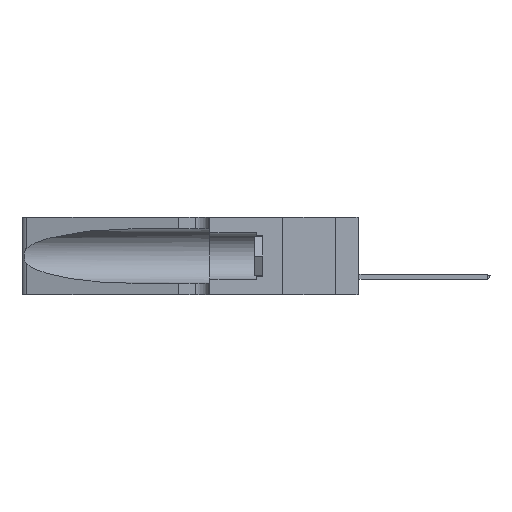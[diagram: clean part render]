
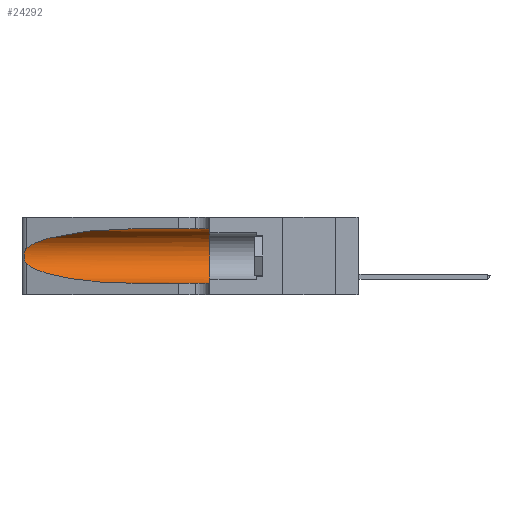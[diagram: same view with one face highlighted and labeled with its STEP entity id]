
A CAD part, left-side view. The second image highlights one B-rep face of the part: STEP entity #24292.
In plain terms, the highlighted cylindrical face has radius 3.308 mm (diameter 6.617 mm), a partial arc.
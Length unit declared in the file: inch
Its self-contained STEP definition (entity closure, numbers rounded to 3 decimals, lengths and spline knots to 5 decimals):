
#578 = ORIENTED_EDGE ( 'NONE', *, *, #11066, .F. ) ;
#1129 = VERTEX_POINT ( 'NONE', #12035 ) ;
#1414 = CARTESIAN_POINT ( 'NONE',  ( 0.25487, 1.22718, 0.14631 ) ) ;
#2001 = EDGE_CURVE ( 'NONE', #14737, #4103, #17094, .T. ) ;
#2032 = ORIENTED_EDGE ( 'NONE', *, *, #13607, .F. ) ;
#2352 = CARTESIAN_POINT ( 'NONE',  ( 0.1305, 0.72297, 0.31525 ) ) ;
#2477 = CARTESIAN_POINT ( 'NONE',  ( 0.1305, 1.61858, 0.31525 ) ) ;
#2659 = CARTESIAN_POINT ( 'NONE',  ( 0.25487, 1.22718, 0.22369 ) ) ;
#2972 = VERTEX_POINT ( 'NONE', #2352 ) ;
#3189 = CARTESIAN_POINT ( 'NONE',  ( 0.25487, 1.22718, 0.22369 ) ) ;
#3365 = CARTESIAN_POINT ( 'NONE',  ( 0.2373, 1.15595, 0.28018 ) ) ;
#3425 = CARTESIAN_POINT ( 'NONE',  ( 0.26075, 1.23896, 0.19203 ) ) ;
#3969 = AXIS2_PLACEMENT_3D ( 'NONE', #17605, #17777, #21797 ) ;
#4103 = VERTEX_POINT ( 'NONE', #18548 ) ;
#4219 = LINE ( 'NONE', #2477, #13924 ) ;
#4576 = EDGE_CURVE ( 'NONE', #2972, #10317, #12386, .T. ) ;
#5140 = CARTESIAN_POINT ( 'NONE',  ( 0.25787, 1.23484, 0.2124 ) ) ;
#5484 = CARTESIAN_POINT ( 'NONE',  ( 0.25487, 1.22718, 0.22369 ) ) ;
#5538 = EDGE_CURVE ( 'NONE', #10317, #14737, #11249, .T. ) ;
#5572 = ORIENTED_EDGE ( 'NONE', *, *, #2001, .T. ) ;
#7021 = ORIENTED_EDGE ( 'NONE', *, *, #15841, .T. ) ;
#7035 = CARTESIAN_POINT ( 'NONE',  ( 0.26017, 1.23833, 0.17102 ) ) ;
#7120 = CARTESIAN_POINT ( 'NONE',  ( 0.26018, 1.23835, 0.19895 ) ) ;
#7374 = CARTESIAN_POINT ( 'NONE',  ( 0.26075, 1.23896, 0.178 ) ) ;
#7436 = CARTESIAN_POINT ( 'NONE',  ( 0.1305, 0.35, 0.05475 ) ) ;
#7580 = FACE_OUTER_BOUND ( 'NONE', #13297, .T. ) ;
#8083 = ORIENTED_EDGE ( 'NONE', *, *, #4576, .T. ) ;
#8667 = LINE ( 'NONE', #12979, #9627 ) ;
#9627 = VECTOR ( 'NONE', #11195, 39.37008 ) ;
#10317 = VERTEX_POINT ( 'NONE', #2659 ) ;
#11066 = EDGE_CURVE ( 'NONE', #2972, #1129, #4219, .T. ) ;
#11195 = DIRECTION ( 'NONE',  ( 0., -1., 0. ) ) ;
#11231 = CARTESIAN_POINT ( 'NONE',  ( 0.25639, 1.23186, 0.15144 ) ) ;
#11249 = B_SPLINE_CURVE_WITH_KNOTS ( 'NONE', 3,
 ( #5484, #19344, #15117, #5140, #11403, #7120, #3425, #7374, #7035, #21347, #11323, #11231, #17424, #1414 ),
 .UNSPECIFIED., .F., .F.,
 ( 4, 2, 2, 2, 2, 2, 4 ),
 ( 0., 0.00027, 0.00053, 0.00107, 0.0016, 0.00187, 0.00214 ),
 .UNSPECIFIED. ) ;
#11283 = ORIENTED_EDGE ( 'NONE', *, *, #5538, .T. ) ;
#11323 = CARTESIAN_POINT ( 'NONE',  ( 0.25789, 1.23486, 0.15765 ) ) ;
#11403 = CARTESIAN_POINT ( 'NONE',  ( 0.25854, 1.2359, 0.20912 ) ) ;
#11491 = CARTESIAN_POINT ( 'NONE',  ( 0.25487, 1.22718, 0.14631 ) ) ;
#12035 = CARTESIAN_POINT ( 'NONE',  ( 0.1305, 0.35, 0.31525 ) ) ;
#12386 =( BOUNDED_CURVE ( )  B_SPLINE_CURVE ( 3, ( #17191, #23134, #3365, #3189 ),
 .UNSPECIFIED., .F., .F. ) 
 B_SPLINE_CURVE_WITH_KNOTS ( ( 4, 4 ),
 ( 1.5708, 2.84003 ),
 .UNSPECIFIED. ) 
 CURVE ( )  GEOMETRIC_REPRESENTATION_ITEM ( )  RATIONAL_B_SPLINE_CURVE ( ( 1., 0.87, 0.87, 1. ) ) 
 REPRESENTATION_ITEM ( '' )  );
#12979 = CARTESIAN_POINT ( 'NONE',  ( 0.1305, 1.61858, 0.05475 ) ) ;
#13297 = EDGE_LOOP ( 'NONE', ( #8083, #11283, #5572, #7021, #2032, #578 ) ) ;
#13532 = CARTESIAN_POINT ( 'NONE',  ( 0.2373, 1.15595, 0.08982 ) ) ;
#13607 = EDGE_CURVE ( 'NONE', #1129, #16348, #18871, .T. ) ;
#13628 = DIRECTION ( 'NONE',  ( 0., 0., -1. ) ) ;
#13924 = VECTOR ( 'NONE', #18210, 39.37008 ) ;
#14737 = VERTEX_POINT ( 'NONE', #22528 ) ;
#15117 = CARTESIAN_POINT ( 'NONE',  ( 0.25639, 1.23184, 0.21858 ) ) ;
#15456 = CARTESIAN_POINT ( 'NONE',  ( 0.1305, 0.72297, 0.05475 ) ) ;
#15540 = CARTESIAN_POINT ( 'NONE',  ( 0.18966, 0.96281, 0.05475 ) ) ;
#15841 = EDGE_CURVE ( 'NONE', #4103, #16348, #8667, .T. ) ;
#16193 = AXIS2_PLACEMENT_3D ( 'NONE', #21184, #17613, #13628 ) ;
#16348 = VERTEX_POINT ( 'NONE', #7436 ) ;
#17094 =( BOUNDED_CURVE ( )  B_SPLINE_CURVE ( 3, ( #11491, #13532, #15540, #15456 ),
 .UNSPECIFIED., .F., .T. ) 
 B_SPLINE_CURVE_WITH_KNOTS ( ( 4, 4 ),
 ( 3.44316, 4.71239 ),
 .UNSPECIFIED. ) 
 CURVE ( )  GEOMETRIC_REPRESENTATION_ITEM ( )  RATIONAL_B_SPLINE_CURVE ( ( 1., 0.87, 0.87, 1. ) ) 
 REPRESENTATION_ITEM ( '' )  );
#17191 = CARTESIAN_POINT ( 'NONE',  ( 0.1305, 0.72297, 0.31525 ) ) ;
#17424 = CARTESIAN_POINT ( 'NONE',  ( 0.25555, 1.22993, 0.14849 ) ) ;
#17605 = CARTESIAN_POINT ( 'NONE',  ( 0.1305, 0.35, 0.185 ) ) ;
#17613 = DIRECTION ( 'NONE',  ( 0., -1., 0. ) ) ;
#17777 = DIRECTION ( 'NONE',  ( 0., 1., 0. ) ) ;
#18210 = DIRECTION ( 'NONE',  ( 0., -1., 0. ) ) ;
#18548 = CARTESIAN_POINT ( 'NONE',  ( 0.1305, 0.72297, 0.05475 ) ) ;
#18871 = CIRCLE ( 'NONE', #3969, 0.13025 ) ;
#19344 = CARTESIAN_POINT ( 'NONE',  ( 0.25555, 1.22994, 0.2215 ) ) ;
#19531 = CYLINDRICAL_SURFACE ( 'NONE', #16193, 0.13025 ) ;
#21184 = CARTESIAN_POINT ( 'NONE',  ( 0.1305, 1.61858, 0.185 ) ) ;
#21347 = CARTESIAN_POINT ( 'NONE',  ( 0.25856, 1.23593, 0.16098 ) ) ;
#21797 = DIRECTION ( 'NONE',  ( 0., 0., 1. ) ) ;
#22528 = CARTESIAN_POINT ( 'NONE',  ( 0.25487, 1.22718, 0.14631 ) ) ;
#23134 = CARTESIAN_POINT ( 'NONE',  ( 0.18966, 0.96281, 0.31525 ) ) ;
#24292 = ADVANCED_FACE ( 'NONE', ( #7580 ), #19531, .F. ) ;
